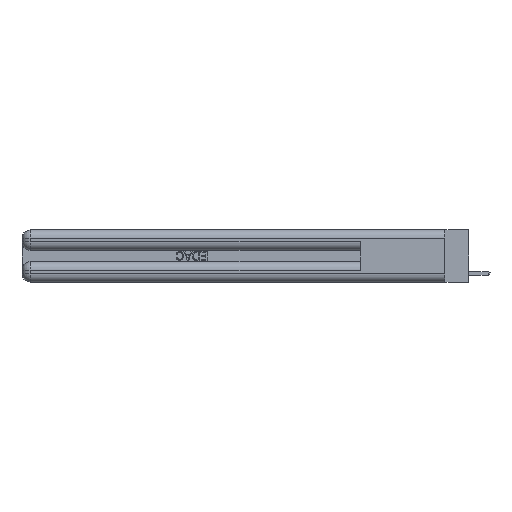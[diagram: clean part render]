
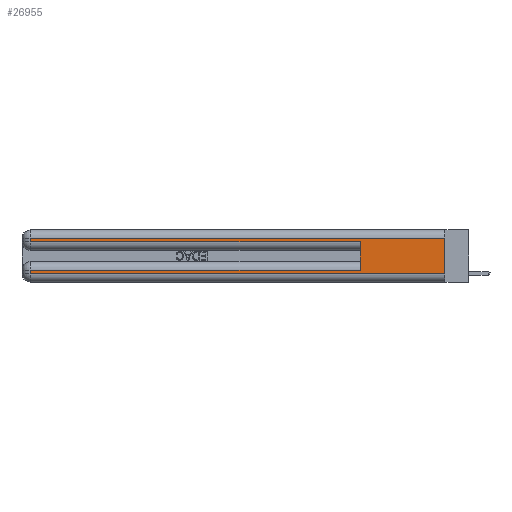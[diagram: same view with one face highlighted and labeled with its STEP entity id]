
A CAD part, left-side view. The second image highlights one B-rep face of the part: STEP entity #26955.
In plain terms, the highlighted planar face has unit normal (-1, 0, 0).
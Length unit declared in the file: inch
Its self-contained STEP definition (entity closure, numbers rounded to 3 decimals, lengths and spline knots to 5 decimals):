
#754 = DIRECTION ( 'NONE',  ( 0., -1., 0. ) ) ;
#857 = LINE ( 'NONE', #26933, #20663 ) ;
#1105 = EDGE_CURVE ( 'NONE', #25961, #5131, #12920, .T. ) ;
#1157 = DIRECTION ( 'NONE',  ( 0., -1., 0. ) ) ;
#1234 = EDGE_CURVE ( 'NONE', #15661, #28124, #857, .T. ) ;
#1902 = CARTESIAN_POINT ( 'NONE',  ( 0., 2.94, 0.31 ) ) ;
#2795 = ORIENTED_EDGE ( 'NONE', *, *, #21566, .T. ) ;
#2828 = LINE ( 'NONE', #28462, #27460 ) ;
#2971 = EDGE_LOOP ( 'NONE', ( #16745, #14141, #2795, #11342, #28816, #17518, #13212, #20662 ) ) ;
#4333 = LINE ( 'NONE', #14855, #15320 ) ;
#5131 = VERTEX_POINT ( 'NONE', #1902 ) ;
#7228 = LINE ( 'NONE', #27777, #20519 ) ;
#7838 = EDGE_CURVE ( 'NONE', #16773, #10037, #4333, .T. ) ;
#8104 = VERTEX_POINT ( 'NONE', #30112 ) ;
#8421 = DIRECTION ( 'NONE',  ( 0., 1., 0. ) ) ;
#8466 = CARTESIAN_POINT ( 'NONE',  ( 0., 0., 0.06 ) ) ;
#8645 = LINE ( 'NONE', #17017, #13806 ) ;
#10037 = VERTEX_POINT ( 'NONE', #8466 ) ;
#10115 = FACE_OUTER_BOUND ( 'NONE', #2971, .T. ) ;
#11117 = VECTOR ( 'NONE', #8421, 39.37008 ) ;
#11342 = ORIENTED_EDGE ( 'NONE', *, *, #1234, .T. ) ;
#11832 = CARTESIAN_POINT ( 'NONE',  ( 0., 2.94, 0.06 ) ) ;
#12266 = DIRECTION ( 'NONE',  ( 0., 0., -1. ) ) ;
#12920 = LINE ( 'NONE', #15103, #11117 ) ;
#13212 = ORIENTED_EDGE ( 'NONE', *, *, #15515, .T. ) ;
#13228 = AXIS2_PLACEMENT_3D ( 'NONE', #28849, #26512, #12266 ) ;
#13386 = DIRECTION ( 'NONE',  ( 0., 0., 1. ) ) ;
#13806 = VECTOR ( 'NONE', #21758, 39.37008 ) ;
#14141 = ORIENTED_EDGE ( 'NONE', *, *, #1105, .T. ) ;
#14266 = EDGE_CURVE ( 'NONE', #8104, #28124, #27168, .T. ) ;
#14562 = VECTOR ( 'NONE', #15951, 39.37008 ) ;
#14855 = CARTESIAN_POINT ( 'NONE',  ( 0., 0., 0.06 ) ) ;
#15103 = CARTESIAN_POINT ( 'NONE',  ( 0., 0., 0.31 ) ) ;
#15320 = VECTOR ( 'NONE', #754, 39.37008 ) ;
#15515 = EDGE_CURVE ( 'NONE', #18462, #16773, #7228, .T. ) ;
#15638 = EDGE_CURVE ( 'NONE', #8104, #18462, #27490, .T. ) ;
#15661 = VERTEX_POINT ( 'NONE', #25623 ) ;
#15743 = VECTOR ( 'NONE', #13386, 39.37008 ) ;
#15787 = EDGE_CURVE ( 'NONE', #25961, #10037, #2828, .T. ) ;
#15914 = CARTESIAN_POINT ( 'NONE',  ( 0., 2.94, 0.085 ) ) ;
#15951 = DIRECTION ( 'NONE',  ( 0., 1., 0. ) ) ;
#16745 = ORIENTED_EDGE ( 'NONE', *, *, #15787, .F. ) ;
#16773 = VERTEX_POINT ( 'NONE', #11832 ) ;
#17017 = CARTESIAN_POINT ( 'NONE',  ( 0., 2.94, 0.37 ) ) ;
#17518 = ORIENTED_EDGE ( 'NONE', *, *, #15638, .T. ) ;
#18462 = VERTEX_POINT ( 'NONE', #15914 ) ;
#19944 = CARTESIAN_POINT ( 'NONE',  ( 0., 0.6, 0.285 ) ) ;
#20519 = VECTOR ( 'NONE', #25516, 39.37008 ) ;
#20662 = ORIENTED_EDGE ( 'NONE', *, *, #7838, .T. ) ;
#20663 = VECTOR ( 'NONE', #1157, 39.37008 ) ;
#20977 = CARTESIAN_POINT ( 'NONE',  ( 0., 0., 0.085 ) ) ;
#21566 = EDGE_CURVE ( 'NONE', #5131, #15661, #8645, .T. ) ;
#21758 = DIRECTION ( 'NONE',  ( 0., 0., -1. ) ) ;
#23483 = DIRECTION ( 'NONE',  ( 0., 0., -1. ) ) ;
#25516 = DIRECTION ( 'NONE',  ( 0., 0., -1. ) ) ;
#25623 = CARTESIAN_POINT ( 'NONE',  ( 0., 2.94, 0.285 ) ) ;
#25961 = VERTEX_POINT ( 'NONE', #29634 ) ;
#26512 = DIRECTION ( 'NONE',  ( 1., 0., 0. ) ) ;
#26933 = CARTESIAN_POINT ( 'NONE',  ( 0., 0., 0.285 ) ) ;
#26955 = ADVANCED_FACE ( 'NONE', ( #10115 ), #28533, .F. ) ;
#27168 = LINE ( 'NONE', #27818, #15743 ) ;
#27460 = VECTOR ( 'NONE', #23483, 39.37008 ) ;
#27490 = LINE ( 'NONE', #20977, #14562 ) ;
#27777 = CARTESIAN_POINT ( 'NONE',  ( 0., 2.94, 0.37 ) ) ;
#27818 = CARTESIAN_POINT ( 'NONE',  ( 0., 0.6, 0.145 ) ) ;
#28124 = VERTEX_POINT ( 'NONE', #19944 ) ;
#28462 = CARTESIAN_POINT ( 'NONE',  ( 0., 0., 0.37 ) ) ;
#28533 = PLANE ( 'NONE',  #13228 ) ;
#28816 = ORIENTED_EDGE ( 'NONE', *, *, #14266, .F. ) ;
#28849 = CARTESIAN_POINT ( 'NONE',  ( 0., 0., 0.37 ) ) ;
#29634 = CARTESIAN_POINT ( 'NONE',  ( 0., 0., 0.31 ) ) ;
#30112 = CARTESIAN_POINT ( 'NONE',  ( 0., 0.6, 0.085 ) ) ;
